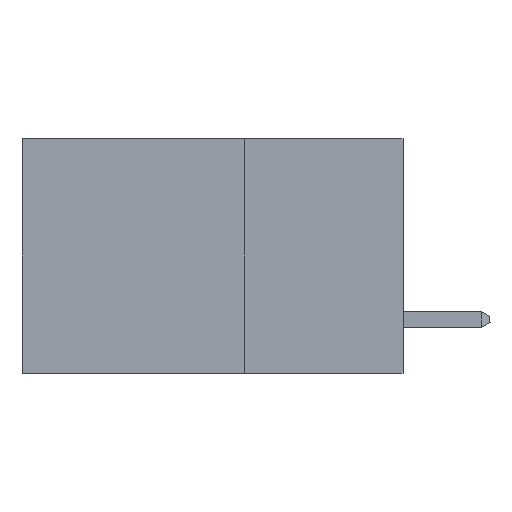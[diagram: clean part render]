
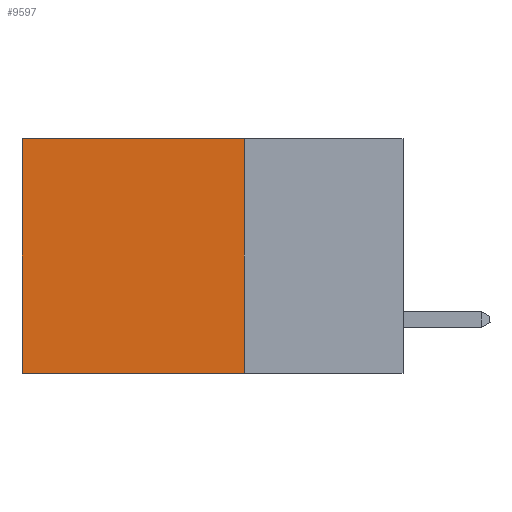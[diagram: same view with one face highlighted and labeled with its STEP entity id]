
A CAD part, left-side view. The second image highlights one B-rep face of the part: STEP entity #9597.
In plain terms, the highlighted planar face has unit normal (-1, 0, 0).
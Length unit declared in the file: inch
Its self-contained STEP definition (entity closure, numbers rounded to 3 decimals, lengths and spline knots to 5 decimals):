
#1876 = LINE ( 'NONE', #2708, #15200 ) ;
#2708 = CARTESIAN_POINT ( 'NONE',  ( 0.2875, 0.25, 0. ) ) ;
#3832 = LINE ( 'NONE', #21504, #9919 ) ;
#4535 = CARTESIAN_POINT ( 'NONE',  ( 0.2875, 0.6, 0. ) ) ;
#4941 = DIRECTION ( 'NONE',  ( 0., 1., 0. ) ) ;
#5044 = VERTEX_POINT ( 'NONE', #21757 ) ;
#5315 = EDGE_CURVE ( 'NONE', #8045, #13040, #6103, .T. ) ;
#6103 = LINE ( 'NONE', #4535, #11393 ) ;
#6198 = CARTESIAN_POINT ( 'NONE',  ( 0.2875, 0.6, -0.37 ) ) ;
#8045 = VERTEX_POINT ( 'NONE', #20407 ) ;
#8716 = ORIENTED_EDGE ( 'NONE', *, *, #9102, .F. ) ;
#9102 = EDGE_CURVE ( 'NONE', #22067, #5044, #1876, .T. ) ;
#9597 = ADVANCED_FACE ( 'NONE', ( #16283 ), #19188, .F. ) ;
#9919 = VECTOR ( 'NONE', #18228, 39.37008 ) ;
#11393 = VECTOR ( 'NONE', #18703, 39.37008 ) ;
#12017 = DIRECTION ( 'NONE',  ( 0., 0., -1. ) ) ;
#13040 = VERTEX_POINT ( 'NONE', #6198 ) ;
#15049 = DIRECTION ( 'NONE',  ( 0., 0., -1. ) ) ;
#15096 = ORIENTED_EDGE ( 'NONE', *, *, #5315, .T. ) ;
#15200 = VECTOR ( 'NONE', #15049, 39.37008 ) ;
#15552 = ORIENTED_EDGE ( 'NONE', *, *, #21972, .F. ) ;
#15649 = CARTESIAN_POINT ( 'NONE',  ( 0.2875, 0.25, 0. ) ) ;
#15882 = ORIENTED_EDGE ( 'NONE', *, *, #17283, .T. ) ;
#16283 = FACE_OUTER_BOUND ( 'NONE', #19082, .T. ) ;
#17283 = EDGE_CURVE ( 'NONE', #22067, #8045, #3832, .T. ) ;
#17577 = CARTESIAN_POINT ( 'NONE',  ( 0.2875, 0.25, -0.37 ) ) ;
#18228 = DIRECTION ( 'NONE',  ( 0., 1., 0. ) ) ;
#18703 = DIRECTION ( 'NONE',  ( 0., 0., -1. ) ) ;
#19082 = EDGE_LOOP ( 'NONE', ( #15096, #15552, #8716, #15882 ) ) ;
#19188 = PLANE ( 'NONE',  #22850 ) ;
#20170 = LINE ( 'NONE', #17577, #22104 ) ;
#20407 = CARTESIAN_POINT ( 'NONE',  ( 0.2875, 0.6, 0. ) ) ;
#21129 = DIRECTION ( 'NONE',  ( 1., 0., 0. ) ) ;
#21363 = CARTESIAN_POINT ( 'NONE',  ( 0.2875, 0.25, 0. ) ) ;
#21504 = CARTESIAN_POINT ( 'NONE',  ( 0.2875, 0.25, 0. ) ) ;
#21757 = CARTESIAN_POINT ( 'NONE',  ( 0.2875, 0.25, -0.37 ) ) ;
#21972 = EDGE_CURVE ( 'NONE', #5044, #13040, #20170, .T. ) ;
#22067 = VERTEX_POINT ( 'NONE', #21363 ) ;
#22104 = VECTOR ( 'NONE', #4941, 39.37008 ) ;
#22850 = AXIS2_PLACEMENT_3D ( 'NONE', #15649, #21129, #12017 ) ;
